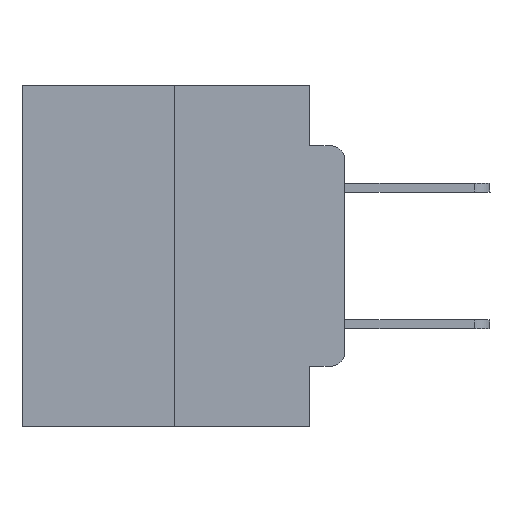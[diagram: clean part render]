
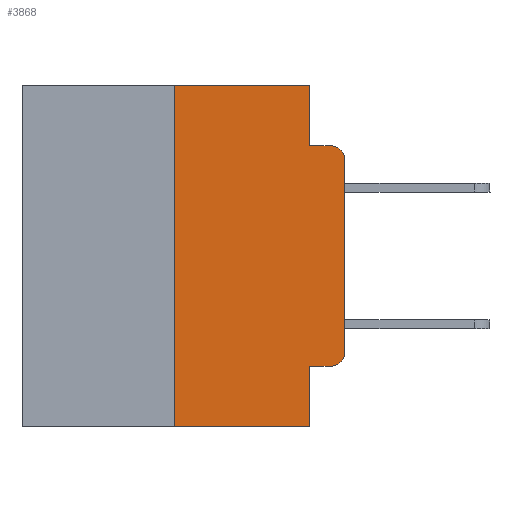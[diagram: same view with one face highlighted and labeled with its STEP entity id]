
A CAD part, left-side view. The second image highlights one B-rep face of the part: STEP entity #3868.
In plain terms, the highlighted planar face has unit normal (-1, 0, 0).
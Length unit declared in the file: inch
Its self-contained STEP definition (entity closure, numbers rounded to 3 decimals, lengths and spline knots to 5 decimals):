
#444 = VERTEX_POINT ( 'NONE', #2620 ) ;
#505 = LINE ( 'NONE', #16214, #19486 ) ;
#745 = DIRECTION ( 'NONE',  ( 0., -1., 0. ) ) ;
#1334 = VERTEX_POINT ( 'NONE', #10388 ) ;
#1915 = VERTEX_POINT ( 'NONE', #23604 ) ;
#2203 = CIRCLE ( 'NONE', #20590, 0.02 ) ;
#2368 = VERTEX_POINT ( 'NONE', #17333 ) ;
#2620 = CARTESIAN_POINT ( 'NONE',  ( 0., 0., -0.3915 ) ) ;
#2821 = VERTEX_POINT ( 'NONE', #6211 ) ;
#3047 = DIRECTION ( 'NONE',  ( 0., 0., -1. ) ) ;
#3098 = EDGE_CURVE ( 'NONE', #11089, #444, #16452, .T. ) ;
#3430 = DIRECTION ( 'NONE',  ( 0., -1., 0. ) ) ;
#3868 = ADVANCED_FACE ( 'NONE', ( #15156 ), #6416, .F. ) ;
#4099 = VERTEX_POINT ( 'NONE', #18966 ) ;
#4288 = AXIS2_PLACEMENT_3D ( 'NONE', #24113, #17282, #15313 ) ;
#4340 = LINE ( 'NONE', #24013, #24918 ) ;
#4939 = CARTESIAN_POINT ( 'NONE',  ( 0., 0.25, 0. ) ) ;
#4964 = DIRECTION ( 'NONE',  ( 0., 0., -1. ) ) ;
#5722 = ORIENTED_EDGE ( 'NONE', *, *, #15695, .T. ) ;
#5777 = VECTOR ( 'NONE', #21233, 39.37008 ) ;
#5940 = VECTOR ( 'NONE', #4964, 39.37008 ) ;
#6100 = EDGE_CURVE ( 'NONE', #10854, #18784, #25292, .T. ) ;
#6211 = CARTESIAN_POINT ( 'NONE',  ( 0., 0., -0.1085 ) ) ;
#6416 = PLANE ( 'NONE',  #26507 ) ;
#6510 = CARTESIAN_POINT ( 'NONE',  ( 0., 0.473, 0. ) ) ;
#6833 = ORIENTED_EDGE ( 'NONE', *, *, #3098, .T. ) ;
#6860 = CARTESIAN_POINT ( 'NONE',  ( 0., 0.051, -0.4115 ) ) ;
#7486 = DIRECTION ( 'NONE',  ( 0., 0., 1. ) ) ;
#7915 = ORIENTED_EDGE ( 'NONE', *, *, #24046, .T. ) ;
#8001 = ORIENTED_EDGE ( 'NONE', *, *, #12185, .F. ) ;
#8597 = CARTESIAN_POINT ( 'NONE',  ( 0., 0.051, 0. ) ) ;
#8666 = DIRECTION ( 'NONE',  ( 0., 0., -1. ) ) ;
#9293 = CARTESIAN_POINT ( 'NONE',  ( 0., 0.051, -0.0885 ) ) ;
#9517 = VERTEX_POINT ( 'NONE', #20558 ) ;
#10244 = EDGE_CURVE ( 'NONE', #18784, #2368, #14965, .T. ) ;
#10388 = CARTESIAN_POINT ( 'NONE',  ( 0., 0.25, -0.5 ) ) ;
#10415 = EDGE_CURVE ( 'NONE', #1334, #10854, #4340, .T. ) ;
#10478 = DIRECTION ( 'NONE',  ( 0., 0., -1. ) ) ;
#10541 = DIRECTION ( 'NONE',  ( 1., 0., 0. ) ) ;
#10854 = VERTEX_POINT ( 'NONE', #4939 ) ;
#11089 = VERTEX_POINT ( 'NONE', #24256 ) ;
#12071 = EDGE_CURVE ( 'NONE', #1334, #1915, #22261, .T. ) ;
#12185 = EDGE_CURVE ( 'NONE', #2368, #9517, #21611, .T. ) ;
#12913 = ORIENTED_EDGE ( 'NONE', *, *, #17882, .T. ) ;
#13489 = ORIENTED_EDGE ( 'NONE', *, *, #12071, .T. ) ;
#14965 = LINE ( 'NONE', #25788, #5940 ) ;
#15073 = ORIENTED_EDGE ( 'NONE', *, *, #10244, .F. ) ;
#15156 = FACE_OUTER_BOUND ( 'NONE', #18769, .T. ) ;
#15313 = DIRECTION ( 'NONE',  ( 0., 0., -1. ) ) ;
#15695 = EDGE_CURVE ( 'NONE', #4099, #11089, #16734, .T. ) ;
#16214 = CARTESIAN_POINT ( 'NONE',  ( 0., 0., 0. ) ) ;
#16452 = CIRCLE ( 'NONE', #4288, 0.02 ) ;
#16734 = LINE ( 'NONE', #6860, #5777 ) ;
#16788 = VECTOR ( 'NONE', #745, 39.37008 ) ;
#17282 = DIRECTION ( 'NONE',  ( -1., 0., 0. ) ) ;
#17333 = CARTESIAN_POINT ( 'NONE',  ( 0., 0.051, -0.0885 ) ) ;
#17343 = DIRECTION ( 'NONE',  ( -1., 0., 0. ) ) ;
#17882 = EDGE_CURVE ( 'NONE', #444, #2821, #505, .T. ) ;
#18769 = EDGE_LOOP ( 'NONE', ( #12913, #7915, #8001, #15073, #23878, #24558, #13489, #18952, #5722, #6833 ) ) ;
#18784 = VERTEX_POINT ( 'NONE', #22715 ) ;
#18952 = ORIENTED_EDGE ( 'NONE', *, *, #26591, .F. ) ;
#18966 = CARTESIAN_POINT ( 'NONE',  ( 0., 0.051, -0.4115 ) ) ;
#19461 = VECTOR ( 'NONE', #10478, 39.37008 ) ;
#19486 = VECTOR ( 'NONE', #20156, 39.37008 ) ;
#19856 = VECTOR ( 'NONE', #26122, 39.37008 ) ;
#19950 = CARTESIAN_POINT ( 'NONE',  ( 0., 0.473, 0. ) ) ;
#20156 = DIRECTION ( 'NONE',  ( 0., 0., 1. ) ) ;
#20558 = CARTESIAN_POINT ( 'NONE',  ( 0., 0.02, -0.0885 ) ) ;
#20590 = AXIS2_PLACEMENT_3D ( 'NONE', #21566, #17343, #3047 ) ;
#21233 = DIRECTION ( 'NONE',  ( 0., -1., 0. ) ) ;
#21566 = CARTESIAN_POINT ( 'NONE',  ( 0., 0.02, -0.1085 ) ) ;
#21611 = LINE ( 'NONE', #9293, #25758 ) ;
#22261 = LINE ( 'NONE', #25344, #16788 ) ;
#22715 = CARTESIAN_POINT ( 'NONE',  ( 0., 0.051, 0. ) ) ;
#23604 = CARTESIAN_POINT ( 'NONE',  ( 0., 0.051, -0.5 ) ) ;
#23878 = ORIENTED_EDGE ( 'NONE', *, *, #6100, .F. ) ;
#24013 = CARTESIAN_POINT ( 'NONE',  ( 0., 0.25, 0. ) ) ;
#24046 = EDGE_CURVE ( 'NONE', #2821, #9517, #2203, .T. ) ;
#24113 = CARTESIAN_POINT ( 'NONE',  ( 0., 0.02, -0.3915 ) ) ;
#24256 = CARTESIAN_POINT ( 'NONE',  ( 0., 0.02, -0.4115 ) ) ;
#24558 = ORIENTED_EDGE ( 'NONE', *, *, #10415, .F. ) ;
#24917 = LINE ( 'NONE', #8597, #19461 ) ;
#24918 = VECTOR ( 'NONE', #7486, 39.37008 ) ;
#25292 = LINE ( 'NONE', #19950, #19856 ) ;
#25344 = CARTESIAN_POINT ( 'NONE',  ( 0., 0.473, -0.5 ) ) ;
#25758 = VECTOR ( 'NONE', #3430, 39.37008 ) ;
#25788 = CARTESIAN_POINT ( 'NONE',  ( 0., 0.051, 0. ) ) ;
#26122 = DIRECTION ( 'NONE',  ( 0., -1., 0. ) ) ;
#26507 = AXIS2_PLACEMENT_3D ( 'NONE', #6510, #10541, #8666 ) ;
#26591 = EDGE_CURVE ( 'NONE', #4099, #1915, #24917, .T. ) ;
